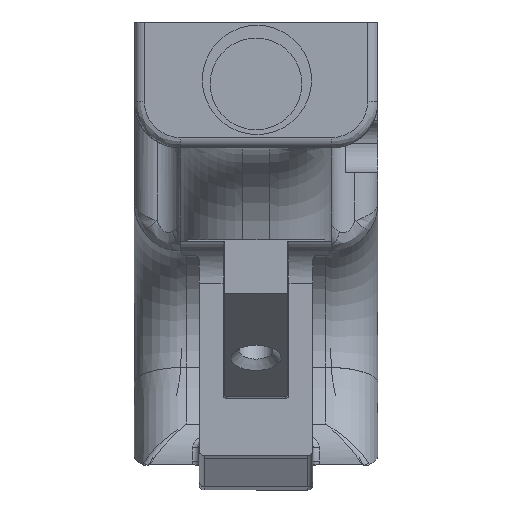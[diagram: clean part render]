
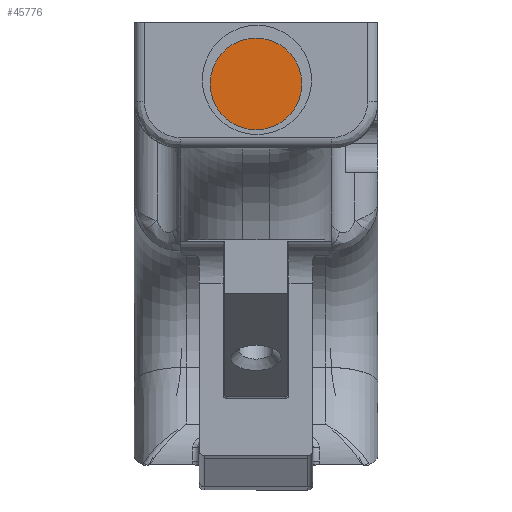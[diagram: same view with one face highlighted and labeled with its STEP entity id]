
A CAD part, left-side view. The second image highlights one B-rep face of the part: STEP entity #45776.
In plain terms, the highlighted planar face has unit normal (-1, 0, 0).
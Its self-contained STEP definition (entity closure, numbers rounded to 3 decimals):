
#14840 = PLANE('',#14841);
#14841 = AXIS2_PLACEMENT_3D('',#14842,#14843,#14844);
#14842 = CARTESIAN_POINT('',(-27.367,102.106,154.638)
  );
#14843 = DIRECTION('',(1.,0.,0.));
#14844 = DIRECTION('',(0.,0.,1.));
#30154 = EDGE_CURVE('',#30155,#30155,#30157,.T.);
#30155 = VERTEX_POINT('',#30156);
#30156 = CARTESIAN_POINT('',(-27.367,110.574,
    147.046));
#30157 = SURFACE_CURVE('',#30158,(#30163,#30170),.PCURVE_S1.);
#30158 = CIRCLE('',#30159,6.985);
#30159 = AXIS2_PLACEMENT_3D('',#30160,#30161,#30162);
#30160 = CARTESIAN_POINT('',(-27.367,110.574,
    154.031));
#30161 = DIRECTION('',(1.,0.,0.));
#30162 = DIRECTION('',(0.,0.,-1.));
#30163 = PCURVE('',#14840,#30164);
#30164 = DEFINITIONAL_REPRESENTATION('',(#30165),#30169);
#30165 = CIRCLE('',#30166,6.985);
#30166 = AXIS2_PLACEMENT_2D('',#30167,#30168);
#30167 = CARTESIAN_POINT('',(-0.608,-8.468));
#30168 = DIRECTION('',(-1.,0.));
#30169 = ( GEOMETRIC_REPRESENTATION_CONTEXT(2) 
PARAMETRIC_REPRESENTATION_CONTEXT() REPRESENTATION_CONTEXT('2D SPACE',''
  ) );
#30170 = PCURVE('',#30171,#30176);
#30171 = PLANE('',#30172);
#30172 = AXIS2_PLACEMENT_3D('',#30173,#30174,#30175);
#30173 = CARTESIAN_POINT('',(-27.367,102.106,154.638)
  );
#30174 = DIRECTION('',(1.,0.,0.));
#30175 = DIRECTION('',(0.,0.,1.));
#30176 = DEFINITIONAL_REPRESENTATION('',(#30177),#30181);
#30177 = CIRCLE('',#30178,6.985);
#30178 = AXIS2_PLACEMENT_2D('',#30179,#30180);
#30179 = CARTESIAN_POINT('',(-0.608,-8.468));
#30180 = DIRECTION('',(-1.,0.));
#30181 = ( GEOMETRIC_REPRESENTATION_CONTEXT(2) 
PARAMETRIC_REPRESENTATION_CONTEXT() REPRESENTATION_CONTEXT('2D SPACE',''
  ) );
#45776 = ADVANCED_FACE('',(#45777),#30171,.F.);
#45777 = FACE_BOUND('',#45778,.F.);
#45778 = EDGE_LOOP('',(#45779));
#45779 = ORIENTED_EDGE('',*,*,#30154,.T.);
